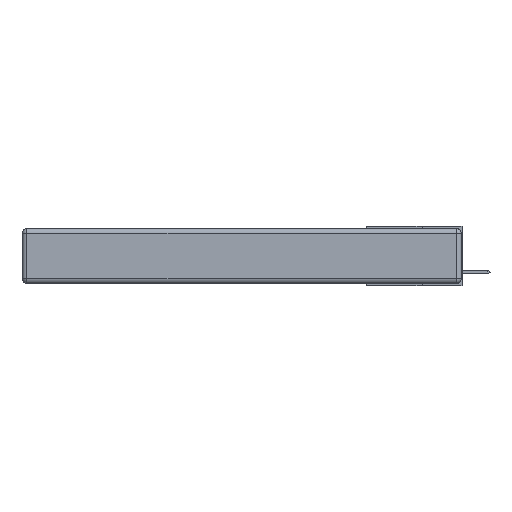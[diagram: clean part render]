
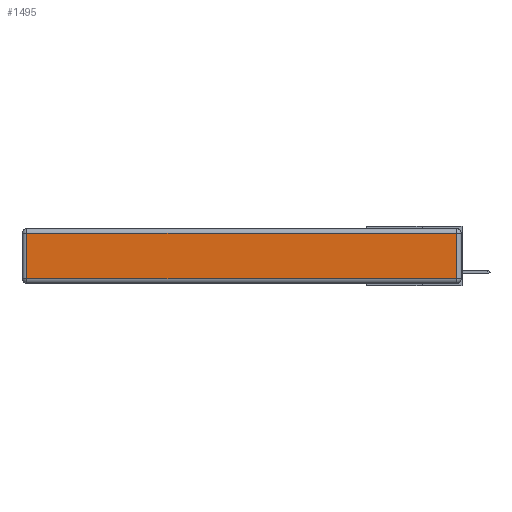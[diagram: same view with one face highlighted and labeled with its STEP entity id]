
A CAD part, left-side view. The second image highlights one B-rep face of the part: STEP entity #1495.
In plain terms, the highlighted planar face has unit normal (-1, 0, 0).
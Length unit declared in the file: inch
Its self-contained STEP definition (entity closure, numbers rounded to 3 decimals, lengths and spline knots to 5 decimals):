
#919 = DIRECTION ( 'NONE',  ( 0., -1., 0. ) ) ;
#965 = CARTESIAN_POINT ( 'NONE',  ( 0., 0., -0.343 ) ) ;
#1366 = DIRECTION ( 'NONE',  ( -1., 0., 0. ) ) ;
#1471 = CARTESIAN_POINT ( 'NONE',  ( 0., 2.72, -0.343 ) ) ;
#1495 = ADVANCED_FACE ( 'NONE', ( #5187 ), #15110, .T. ) ;
#1589 = EDGE_CURVE ( 'NONE', #23198, #10275, #16640, .T. ) ;
#2744 = CARTESIAN_POINT ( 'NONE',  ( 0., 0.03, -0.03 ) ) ;
#2778 = DIRECTION ( 'NONE',  ( 0., 0., 1. ) ) ;
#3396 = EDGE_CURVE ( 'NONE', #11507, #23198, #6141, .T. ) ;
#4647 = ORIENTED_EDGE ( 'NONE', *, *, #1589, .T. ) ;
#5187 = FACE_OUTER_BOUND ( 'NONE', #20576, .T. ) ;
#5730 = CARTESIAN_POINT ( 'NONE',  ( 0., 2.72, -0.313 ) ) ;
#5869 = ORIENTED_EDGE ( 'NONE', *, *, #27968, .T. ) ;
#6141 = LINE ( 'NONE', #28031, #12244 ) ;
#7985 = VECTOR ( 'NONE', #919, 39.37008 ) ;
#8068 = DIRECTION ( 'NONE',  ( 0., 1., 0. ) ) ;
#10275 = VERTEX_POINT ( 'NONE', #29205 ) ;
#11507 = VERTEX_POINT ( 'NONE', #14861 ) ;
#12244 = VECTOR ( 'NONE', #2778, 39.37008 ) ;
#12672 = LINE ( 'NONE', #1471, #27091 ) ;
#14861 = CARTESIAN_POINT ( 'NONE',  ( 0., 0.03, -0.313 ) ) ;
#15110 = PLANE ( 'NONE',  #24172 ) ;
#16121 = ORIENTED_EDGE ( 'NONE', *, *, #20789, .T. ) ;
#16640 = LINE ( 'NONE', #28648, #23127 ) ;
#17543 = DIRECTION ( 'NONE',  ( 0., 0., -1. ) ) ;
#20576 = EDGE_LOOP ( 'NONE', ( #5869, #21096, #4647, #16121 ) ) ;
#20789 = EDGE_CURVE ( 'NONE', #10275, #24751, #12672, .T. ) ;
#21096 = ORIENTED_EDGE ( 'NONE', *, *, #3396, .T. ) ;
#21468 = CARTESIAN_POINT ( 'NONE',  ( 0., 0., -0.313 ) ) ;
#23127 = VECTOR ( 'NONE', #8068, 39.37008 ) ;
#23198 = VERTEX_POINT ( 'NONE', #2744 ) ;
#24172 = AXIS2_PLACEMENT_3D ( 'NONE', #965, #1366, #26458 ) ;
#24751 = VERTEX_POINT ( 'NONE', #5730 ) ;
#26311 = LINE ( 'NONE', #21468, #7985 ) ;
#26458 = DIRECTION ( 'NONE',  ( 0., 0., 1. ) ) ;
#27091 = VECTOR ( 'NONE', #17543, 39.37008 ) ;
#27968 = EDGE_CURVE ( 'NONE', #24751, #11507, #26311, .T. ) ;
#28031 = CARTESIAN_POINT ( 'NONE',  ( 0., 0.03, -0.343 ) ) ;
#28648 = CARTESIAN_POINT ( 'NONE',  ( 0., 2.75, -0.03 ) ) ;
#29205 = CARTESIAN_POINT ( 'NONE',  ( 0., 2.72, -0.03 ) ) ;
